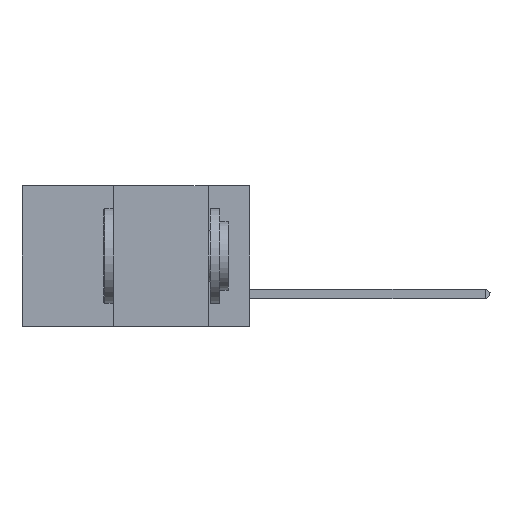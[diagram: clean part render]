
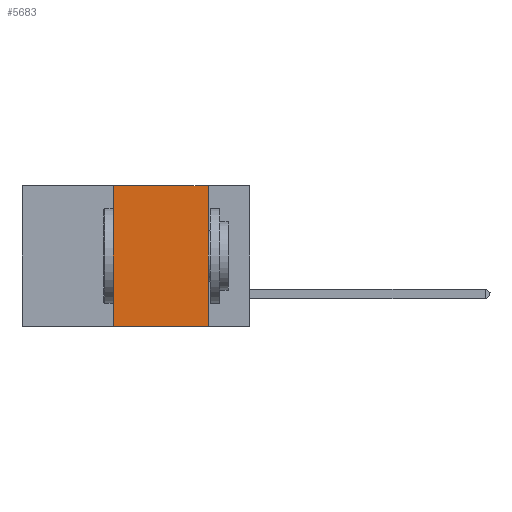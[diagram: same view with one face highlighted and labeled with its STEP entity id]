
A CAD part, left-side view. The second image highlights one B-rep face of the part: STEP entity #5683.
In plain terms, the highlighted planar face has unit normal (-1, 0, 0).
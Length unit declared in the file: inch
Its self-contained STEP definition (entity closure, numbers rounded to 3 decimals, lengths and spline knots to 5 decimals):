
#818 = VECTOR ( 'NONE', #3998, 39.37008 ) ;
#1048 = CARTESIAN_POINT ( 'NONE',  ( 0., 0.6, 0. ) ) ;
#1150 = DIRECTION ( 'NONE',  ( 1., 0., 0. ) ) ;
#2577 = CARTESIAN_POINT ( 'NONE',  ( 0., 0.6, -0.37 ) ) ;
#3056 = DIRECTION ( 'NONE',  ( 0., 0., 1. ) ) ;
#3460 = CARTESIAN_POINT ( 'NONE',  ( 0., 0.36, -0.37 ) ) ;
#3998 = DIRECTION ( 'NONE',  ( 0., -1., 0. ) ) ;
#4925 = CARTESIAN_POINT ( 'NONE',  ( 0., 0.11, -0.37 ) ) ;
#5683 = ADVANCED_FACE ( 'NONE', ( #10619 ), #29570, .F. ) ;
#6589 = DIRECTION ( 'NONE',  ( 0., 0., -1. ) ) ;
#6762 = CARTESIAN_POINT ( 'NONE',  ( 0., 0.36, 0. ) ) ;
#6864 = LINE ( 'NONE', #29328, #21388 ) ;
#7137 = ORIENTED_EDGE ( 'NONE', *, *, #8981, .F. ) ;
#7165 = EDGE_CURVE ( 'NONE', #22514, #15514, #6864, .T. ) ;
#8981 = EDGE_CURVE ( 'NONE', #32650, #22514, #12044, .T. ) ;
#9122 = ORIENTED_EDGE ( 'NONE', *, *, #7165, .F. ) ;
#9312 = VERTEX_POINT ( 'NONE', #3460 ) ;
#10619 = FACE_OUTER_BOUND ( 'NONE', #17572, .T. ) ;
#10820 = LINE ( 'NONE', #2577, #29442 ) ;
#11850 = DIRECTION ( 'NONE',  ( 0., -1., 0. ) ) ;
#12044 = LINE ( 'NONE', #1048, #818 ) ;
#14332 = EDGE_CURVE ( 'NONE', #9312, #32650, #14507, .T. ) ;
#14507 = LINE ( 'NONE', #16533, #29753 ) ;
#15514 = VERTEX_POINT ( 'NONE', #4925 ) ;
#16261 = DIRECTION ( 'NONE',  ( 0., 0., -1. ) ) ;
#16344 = ORIENTED_EDGE ( 'NONE', *, *, #14332, .F. ) ;
#16345 = ORIENTED_EDGE ( 'NONE', *, *, #26914, .T. ) ;
#16533 = CARTESIAN_POINT ( 'NONE',  ( 0., 0.36, 0. ) ) ;
#17572 = EDGE_LOOP ( 'NONE', ( #9122, #7137, #16344, #16345 ) ) ;
#19094 = CARTESIAN_POINT ( 'NONE',  ( 0., 0.6, 0. ) ) ;
#20915 = CARTESIAN_POINT ( 'NONE',  ( 0., 0.11, 0. ) ) ;
#21388 = VECTOR ( 'NONE', #16261, 39.37008 ) ;
#22514 = VERTEX_POINT ( 'NONE', #20915 ) ;
#24218 = AXIS2_PLACEMENT_3D ( 'NONE', #19094, #1150, #6589 ) ;
#26914 = EDGE_CURVE ( 'NONE', #9312, #15514, #10820, .T. ) ;
#29328 = CARTESIAN_POINT ( 'NONE',  ( 0., 0.11, 0. ) ) ;
#29442 = VECTOR ( 'NONE', #11850, 39.37008 ) ;
#29570 = PLANE ( 'NONE',  #24218 ) ;
#29753 = VECTOR ( 'NONE', #3056, 39.37008 ) ;
#32650 = VERTEX_POINT ( 'NONE', #6762 ) ;
